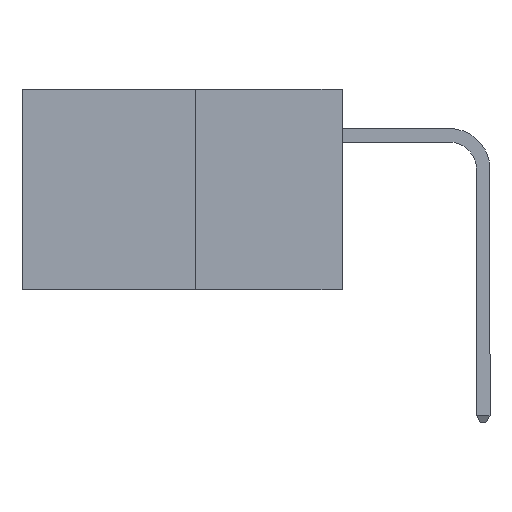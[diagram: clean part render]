
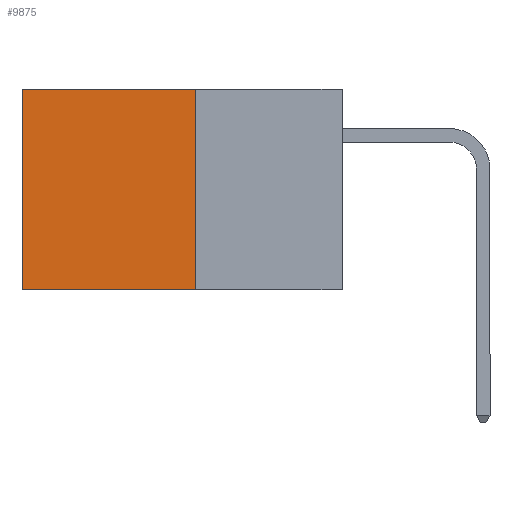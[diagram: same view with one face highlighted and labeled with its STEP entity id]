
A CAD part, left-side view. The second image highlights one B-rep face of the part: STEP entity #9875.
In plain terms, the highlighted planar face has unit normal (-1, 0, 0).
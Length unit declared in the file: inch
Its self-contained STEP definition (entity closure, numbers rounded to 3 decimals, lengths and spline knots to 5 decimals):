
#208 = VERTEX_POINT ( 'NONE', #11364 ) ;
#707 = DIRECTION ( 'NONE',  ( 0., 1., 0. ) ) ;
#955 = VECTOR ( 'NONE', #17829, 39.37008 ) ;
#1583 = LINE ( 'NONE', #14694, #9290 ) ;
#1664 = CARTESIAN_POINT ( 'NONE',  ( 0.277, 0.27, -0.37 ) ) ;
#1805 = CARTESIAN_POINT ( 'NONE',  ( 0.277, 0.27, 0. ) ) ;
#2293 = EDGE_CURVE ( 'NONE', #19197, #13240, #5274, .T. ) ;
#2361 = LINE ( 'NONE', #10934, #10041 ) ;
#2706 = EDGE_CURVE ( 'NONE', #208, #5914, #1583, .T. ) ;
#3252 = DIRECTION ( 'NONE',  ( 0., 0., -1. ) ) ;
#5172 = DIRECTION ( 'NONE',  ( 0., 1., 0. ) ) ;
#5274 = LINE ( 'NONE', #1805, #12815 ) ;
#5910 = CARTESIAN_POINT ( 'NONE',  ( 0.277, 0.59, -0.37 ) ) ;
#5914 = VERTEX_POINT ( 'NONE', #7353 ) ;
#6538 = CARTESIAN_POINT ( 'NONE',  ( 0.277, 0.27, 0. ) ) ;
#7353 = CARTESIAN_POINT ( 'NONE',  ( 0.277, 0.59, -0.37 ) ) ;
#7696 = EDGE_LOOP ( 'NONE', ( #15645, #11992, #16139, #15942 ) ) ;
#9290 = VECTOR ( 'NONE', #707, 39.37008 ) ;
#9875 = ADVANCED_FACE ( 'NONE', ( #12139 ), #13763, .F. ) ;
#10041 = VECTOR ( 'NONE', #12415, 39.37008 ) ;
#10934 = CARTESIAN_POINT ( 'NONE',  ( 0.277, 0.27, -0.37 ) ) ;
#11364 = CARTESIAN_POINT ( 'NONE',  ( 0.277, 0.27, -0.37 ) ) ;
#11992 = ORIENTED_EDGE ( 'NONE', *, *, #2706, .F. ) ;
#12139 = FACE_OUTER_BOUND ( 'NONE', #7696, .T. ) ;
#12336 = DIRECTION ( 'NONE',  ( 1., 0., 0. ) ) ;
#12415 = DIRECTION ( 'NONE',  ( 0., 0., -1. ) ) ;
#12815 = VECTOR ( 'NONE', #5172, 39.37008 ) ;
#13240 = VERTEX_POINT ( 'NONE', #14346 ) ;
#13763 = PLANE ( 'NONE',  #14468 ) ;
#14346 = CARTESIAN_POINT ( 'NONE',  ( 0.277, 0.59, 0. ) ) ;
#14468 = AXIS2_PLACEMENT_3D ( 'NONE', #1664, #12336, #3252 ) ;
#14694 = CARTESIAN_POINT ( 'NONE',  ( 0.277, 0.27, -0.37 ) ) ;
#15645 = ORIENTED_EDGE ( 'NONE', *, *, #16322, .T. ) ;
#15942 = ORIENTED_EDGE ( 'NONE', *, *, #2293, .T. ) ;
#16139 = ORIENTED_EDGE ( 'NONE', *, *, #18571, .F. ) ;
#16322 = EDGE_CURVE ( 'NONE', #13240, #5914, #16989, .T. ) ;
#16989 = LINE ( 'NONE', #5910, #955 ) ;
#17829 = DIRECTION ( 'NONE',  ( 0., 0., -1. ) ) ;
#18571 = EDGE_CURVE ( 'NONE', #19197, #208, #2361, .T. ) ;
#19197 = VERTEX_POINT ( 'NONE', #6538 ) ;
